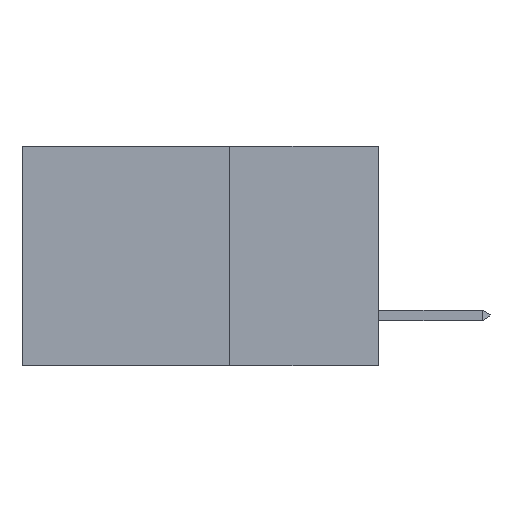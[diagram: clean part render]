
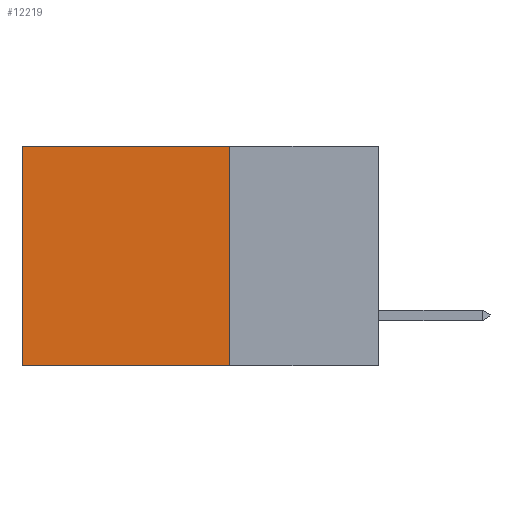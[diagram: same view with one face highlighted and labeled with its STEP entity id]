
A CAD part, left-side view. The second image highlights one B-rep face of the part: STEP entity #12219.
In plain terms, the highlighted planar face has unit normal (-1, 0, 0).
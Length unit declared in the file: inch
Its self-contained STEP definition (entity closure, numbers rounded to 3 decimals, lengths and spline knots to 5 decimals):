
#135 = CARTESIAN_POINT ( 'NONE',  ( 0.298, 0.25, 0. ) ) ;
#463 = EDGE_CURVE ( 'NONE', #6537, #5777, #10312, .T. ) ;
#581 = VERTEX_POINT ( 'NONE', #14895 ) ;
#1654 = LINE ( 'NONE', #2495, #4399 ) ;
#2005 = VECTOR ( 'NONE', #7736, 39.37008 ) ;
#2046 = EDGE_LOOP ( 'NONE', ( #17777, #4207, #9231, #14628 ) ) ;
#2495 = CARTESIAN_POINT ( 'NONE',  ( 0.298, 0.6, 0. ) ) ;
#2870 = CARTESIAN_POINT ( 'NONE',  ( 0.298, 0.25, 0. ) ) ;
#3398 = VECTOR ( 'NONE', #3926, 39.37008 ) ;
#3926 = DIRECTION ( 'NONE',  ( 0., 1., 0. ) ) ;
#4207 = ORIENTED_EDGE ( 'NONE', *, *, #463, .F. ) ;
#4350 = LINE ( 'NONE', #135, #15303 ) ;
#4399 = VECTOR ( 'NONE', #15234, 39.37008 ) ;
#4801 = CARTESIAN_POINT ( 'NONE',  ( 0.298, 0.25, 0. ) ) ;
#5030 = EDGE_CURVE ( 'NONE', #18682, #5777, #1654, .T. ) ;
#5489 = CARTESIAN_POINT ( 'NONE',  ( 0.298, 0.25, -0.37 ) ) ;
#5777 = VERTEX_POINT ( 'NONE', #8758 ) ;
#6537 = VERTEX_POINT ( 'NONE', #13506 ) ;
#7073 = LINE ( 'NONE', #4801, #2005 ) ;
#7736 = DIRECTION ( 'NONE',  ( 0., 1., 0. ) ) ;
#8758 = CARTESIAN_POINT ( 'NONE',  ( 0.298, 0.6, -0.37 ) ) ;
#8763 = FACE_OUTER_BOUND ( 'NONE', #2046, .T. ) ;
#8857 = DIRECTION ( 'NONE',  ( 1., 0., 0. ) ) ;
#9231 = ORIENTED_EDGE ( 'NONE', *, *, #13504, .F. ) ;
#10312 = LINE ( 'NONE', #5489, #3398 ) ;
#10928 = CARTESIAN_POINT ( 'NONE',  ( 0.298, 0.6, 0. ) ) ;
#12219 = ADVANCED_FACE ( 'NONE', ( #8763 ), #17614, .F. ) ;
#13504 = EDGE_CURVE ( 'NONE', #581, #6537, #4350, .T. ) ;
#13506 = CARTESIAN_POINT ( 'NONE',  ( 0.298, 0.25, -0.37 ) ) ;
#14628 = ORIENTED_EDGE ( 'NONE', *, *, #14786, .T. ) ;
#14780 = DIRECTION ( 'NONE',  ( 0., 0., -1. ) ) ;
#14786 = EDGE_CURVE ( 'NONE', #581, #18682, #7073, .T. ) ;
#14895 = CARTESIAN_POINT ( 'NONE',  ( 0.298, 0.25, 0. ) ) ;
#15234 = DIRECTION ( 'NONE',  ( 0., 0., -1. ) ) ;
#15303 = VECTOR ( 'NONE', #16273, 39.37008 ) ;
#15589 = AXIS2_PLACEMENT_3D ( 'NONE', #2870, #8857, #14780 ) ;
#16273 = DIRECTION ( 'NONE',  ( 0., 0., -1. ) ) ;
#17614 = PLANE ( 'NONE',  #15589 ) ;
#17777 = ORIENTED_EDGE ( 'NONE', *, *, #5030, .T. ) ;
#18682 = VERTEX_POINT ( 'NONE', #10928 ) ;
